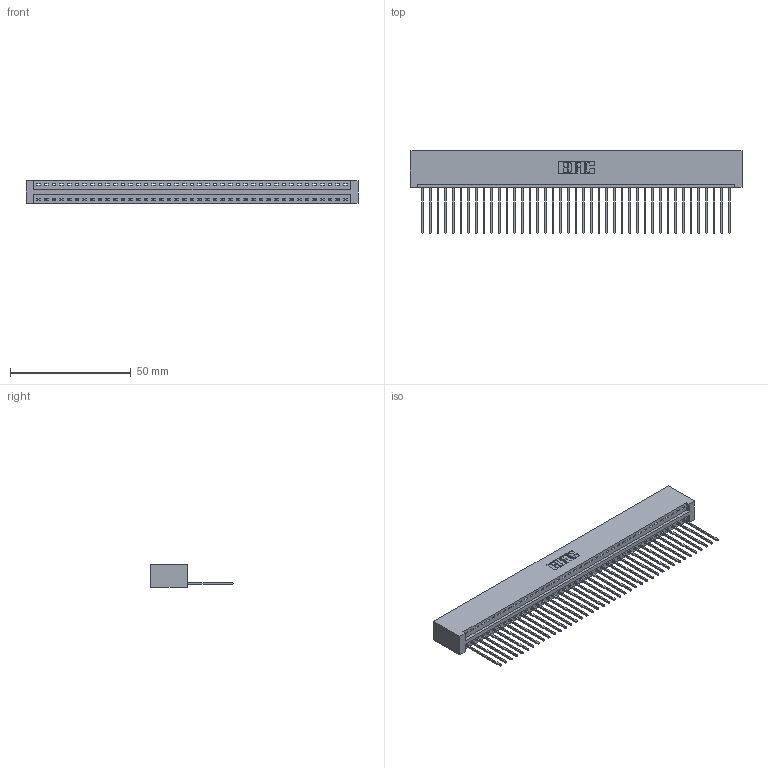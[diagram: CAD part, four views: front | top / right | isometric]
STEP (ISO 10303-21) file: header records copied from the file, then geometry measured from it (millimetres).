
FILE_DESCRIPTION (( 'STEP AP203' ), '1' );
FILE_NAME ('396-041-541-101.STEP', '2019-10-27T21:12:12', ( '' ), ( '' ), 'SwSTEP 2.0', 'SolidWorks 2016', '' );
FILE_SCHEMA (( 'CONFIG_CONTROL_DESIGN' ));
Length unit declared in the file: inch
Products named in the file (3): 346 Part_No Mounting Lugs; 345-292-001_345-293-141; 396-041-541-101
Assembly tree (42 placements, depth 2):
  396-041-541-101
    346 Part_No Mounting Lugs
    345-292-001_345-293-141  x41
Bounding box: 137.41 x 34.29 x 9.4 mm (x, y, z)
Volume: 13831.4 mm3; surface area: 18160 mm2
Topology: 42 solids, 42 shells, 2492 faces, 7521 edges, 4958 vertices
Faces by surface type: plane 1712, cylinder 780
Entity records: 25321 total; most frequent: CARTESIAN_POINT 4347, ORIENTED_EDGE 4322, DIRECTION 3831, EDGE_CURVE 2161, VECTOR 1873, LINE 1873, VERTEX_POINT 1438, AXIS2_PLACEMENT_3D 979
